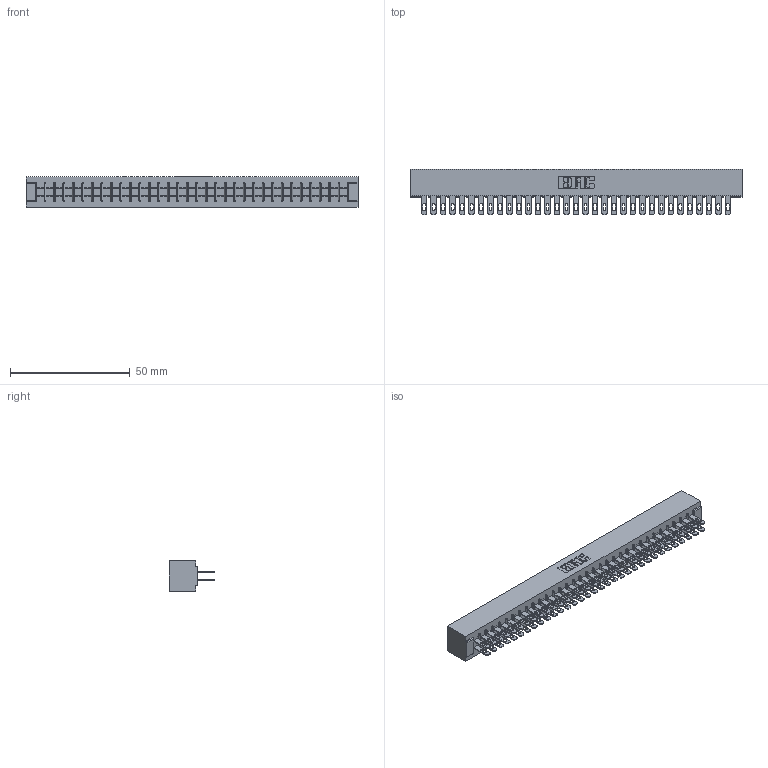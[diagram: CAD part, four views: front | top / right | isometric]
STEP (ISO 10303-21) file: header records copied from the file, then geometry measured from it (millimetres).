
FILE_DESCRIPTION (( 'STEP AP203' ), '1' );
FILE_NAME ('355-066-500-501.STEP', '2019-09-12T15:25:22', ( '' ), ( '' ), 'SwSTEP 2.0', 'SolidWorks 2016', '' );
FILE_SCHEMA (( 'CONFIG_CONTROL_DESIGN' ));
Length unit declared in the file: inch
Products named in the file (3): 305 Part_No Mounting; 305-290-001_500; 355-066-500-501
Assembly tree (67 placements, depth 2):
  355-066-500-501
    305 Part_No Mounting
    305-290-001_500  x66
Bounding box: 138.63 x 18.85 x 12.7 mm (x, y, z)
Volume: 14640.4 mm3; surface area: 20850.7 mm2
Topology: 67 solids, 67 shells, 3408 faces, 9763 edges, 6330 vertices
Faces by surface type: plane 1912, cylinder 1364, sphere 132
Entity records: 36570 total; most frequent: CARTESIAN_POINT 6049, ORIENTED_EDGE 6002, DIRECTION 5859, EDGE_CURVE 3001, LINE 2419, VECTOR 2419, VERTEX_POINT 1910, AXIS2_PLACEMENT_3D 1720
